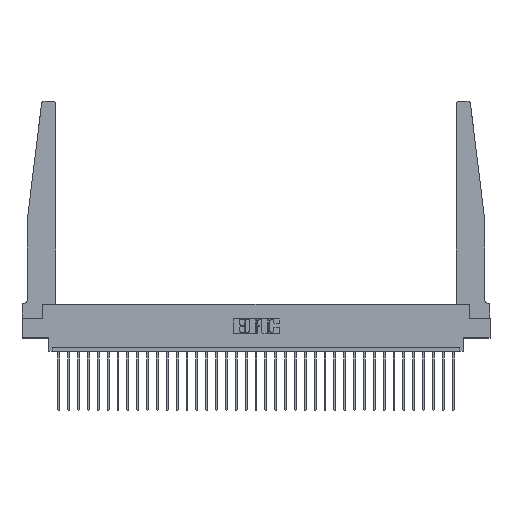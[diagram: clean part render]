
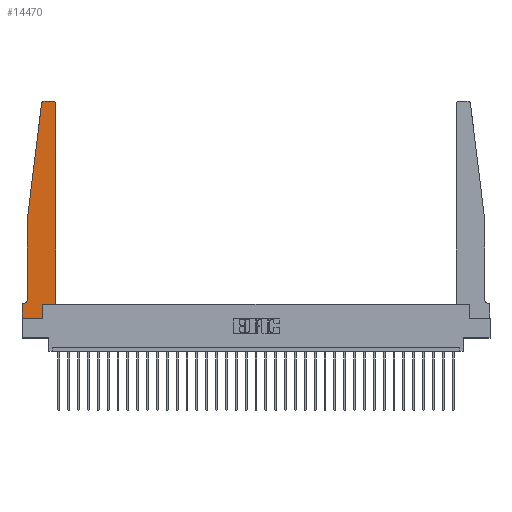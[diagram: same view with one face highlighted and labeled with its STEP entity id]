
A CAD part, top view. The second image highlights one B-rep face of the part: STEP entity #14470.
In plain terms, the highlighted planar face has unit normal (0, 0, 1).
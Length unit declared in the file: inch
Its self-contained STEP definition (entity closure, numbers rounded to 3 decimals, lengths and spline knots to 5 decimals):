
#335 = LINE ( 'NONE', #29155, #5157 ) ;
#478 = VECTOR ( 'NONE', #7500, 39.37008 ) ;
#1019 = VERTEX_POINT ( 'NONE', #19971 ) ;
#2128 = AXIS2_PLACEMENT_3D ( 'NONE', #2731, #24211, #10198 ) ;
#2588 = VERTEX_POINT ( 'NONE', #17972 ) ;
#2600 = DIRECTION ( 'NONE',  ( 0., 0., 1. ) ) ;
#2729 = CARTESIAN_POINT ( 'NONE',  ( 0.425, 0.18, 0.37 ) ) ;
#2731 = CARTESIAN_POINT ( 'NONE',  ( 0.015, 0.2375, 0.37 ) ) ;
#3383 = CARTESIAN_POINT ( 'NONE',  ( 0., 0., 0.37 ) ) ;
#3421 = VECTOR ( 'NONE', #9044, 39.37008 ) ;
#3777 = CARTESIAN_POINT ( 'NONE',  ( 0., 0., 0.37 ) ) ;
#4061 = DIRECTION ( 'NONE',  ( 0., -1., 0. ) ) ;
#4293 = LINE ( 'NONE', #29822, #13118 ) ;
#4560 = EDGE_CURVE ( 'NONE', #19507, #29272, #4293, .T. ) ;
#5157 = VECTOR ( 'NONE', #5846, 39.37008 ) ;
#5846 = DIRECTION ( 'NONE',  ( 0., 1., 0. ) ) ;
#5868 = EDGE_CURVE ( 'NONE', #1019, #19081, #28846, .T. ) ;
#5870 = AXIS2_PLACEMENT_3D ( 'NONE', #26339, #17080, #26533 ) ;
#6393 = EDGE_CURVE ( 'NONE', #19081, #13151, #6403, .T. ) ;
#6403 = LINE ( 'NONE', #25717, #3421 ) ;
#7042 = FACE_OUTER_BOUND ( 'NONE', #27884, .T. ) ;
#7092 = ORIENTED_EDGE ( 'NONE', *, *, #30292, .T. ) ;
#7118 = VECTOR ( 'NONE', #29553, 39.37008 ) ;
#7170 = VERTEX_POINT ( 'NONE', #22088 ) ;
#7500 = DIRECTION ( 'NONE',  ( -0.122, -0.992, 0. ) ) ;
#9044 = DIRECTION ( 'NONE',  ( -1., 0., 0. ) ) ;
#9085 = VECTOR ( 'NONE', #27528, 39.37008 ) ;
#9209 = CARTESIAN_POINT ( 'NONE',  ( 0.425, 0.18, 0.37 ) ) ;
#9689 = DIRECTION ( 'NONE',  ( 1., 0., 0. ) ) ;
#10198 = DIRECTION ( 'NONE',  ( -1., 0., 0. ) ) ;
#10376 = ORIENTED_EDGE ( 'NONE', *, *, #4560, .T. ) ;
#10583 = CIRCLE ( 'NONE', #14198, 0.03 ) ;
#10783 = CARTESIAN_POINT ( 'NONE',  ( 0.395, 2.75, 0.37 ) ) ;
#11486 = CARTESIAN_POINT ( 'NONE',  ( 0., 0., 0.37 ) ) ;
#11532 = LINE ( 'NONE', #15961, #18524 ) ;
#11783 = DIRECTION ( 'NONE',  ( 1., 0., 0. ) ) ;
#11981 = CARTESIAN_POINT ( 'NONE',  ( 0.395, 2.72, 0.37 ) ) ;
#12432 = VERTEX_POINT ( 'NONE', #9209 ) ;
#12606 = LINE ( 'NONE', #20045, #7118 ) ;
#13028 = EDGE_CURVE ( 'NONE', #2588, #16459, #335, .T. ) ;
#13118 = VECTOR ( 'NONE', #18357, 39.37008 ) ;
#13151 = VERTEX_POINT ( 'NONE', #30263 ) ;
#13926 = VERTEX_POINT ( 'NONE', #3777 ) ;
#14198 = AXIS2_PLACEMENT_3D ( 'NONE', #11981, #2600, #11783 ) ;
#14470 = ADVANCED_FACE ( 'NONE', ( #7042 ), #17662, .T. ) ;
#14613 = VECTOR ( 'NONE', #9689, 39.37008 ) ;
#14833 = VERTEX_POINT ( 'NONE', #28486 ) ;
#15491 = DIRECTION ( 'NONE',  ( 1., 0., 0. ) ) ;
#15695 = CARTESIAN_POINT ( 'NONE',  ( 0., 0.1875, 0.37 ) ) ;
#15961 = CARTESIAN_POINT ( 'NONE',  ( 0.425, 0.18, 0.37 ) ) ;
#16459 = VERTEX_POINT ( 'NONE', #22634 ) ;
#16899 = ORIENTED_EDGE ( 'NONE', *, *, #5868, .T. ) ;
#17080 = DIRECTION ( 'NONE',  ( 0., 0., 1. ) ) ;
#17412 = EDGE_CURVE ( 'NONE', #16459, #12432, #25961, .T. ) ;
#17662 = PLANE ( 'NONE',  #23762 ) ;
#17806 = CIRCLE ( 'NONE', #5870, 0.03 ) ;
#17830 = EDGE_CURVE ( 'NONE', #13151, #13926, #22650, .T. ) ;
#17872 = EDGE_CURVE ( 'NONE', #14833, #19507, #10583, .T. ) ;
#17972 = CARTESIAN_POINT ( 'NONE',  ( 0.2605, 0., 0.37 ) ) ;
#18357 = DIRECTION ( 'NONE',  ( -1., 0., 0. ) ) ;
#18524 = VECTOR ( 'NONE', #30218, 39.37008 ) ;
#18651 = VECTOR ( 'NONE', #4061, 39.37008 ) ;
#18838 = CARTESIAN_POINT ( 'NONE',  ( 0.015, 0.1875, 0.37 ) ) ;
#19044 = EDGE_CURVE ( 'NONE', #7170, #26273, #24016, .T. ) ;
#19081 = VERTEX_POINT ( 'NONE', #18838 ) ;
#19507 = VERTEX_POINT ( 'NONE', #10783 ) ;
#19910 = DIRECTION ( 'NONE',  ( 0., 0., 1. ) ) ;
#19971 = CARTESIAN_POINT ( 'NONE',  ( 0.065, 0.2375, 0.37 ) ) ;
#20045 = CARTESIAN_POINT ( 'NONE',  ( 0.065, 1.25, 0.37 ) ) ;
#20674 = ORIENTED_EDGE ( 'NONE', *, *, #6393, .T. ) ;
#21165 = ORIENTED_EDGE ( 'NONE', *, *, #13028, .T. ) ;
#21500 = ORIENTED_EDGE ( 'NONE', *, *, #19044, .T. ) ;
#22088 = CARTESIAN_POINT ( 'NONE',  ( 0.24675, 2.72367, 0.37 ) ) ;
#22130 = ORIENTED_EDGE ( 'NONE', *, *, #17412, .T. ) ;
#22634 = CARTESIAN_POINT ( 'NONE',  ( 0.2605, 0.18, 0.37 ) ) ;
#22650 = LINE ( 'NONE', #11486, #18651 ) ;
#22663 = LINE ( 'NONE', #3383, #9085 ) ;
#23080 = ORIENTED_EDGE ( 'NONE', *, *, #25417, .T. ) ;
#23214 = ORIENTED_EDGE ( 'NONE', *, *, #28178, .T. ) ;
#23464 = CARTESIAN_POINT ( 'NONE',  ( 0.065, 1.25, 0.37 ) ) ;
#23710 = CARTESIAN_POINT ( 'NONE',  ( 0.065, 1.25, 0.37 ) ) ;
#23721 = ORIENTED_EDGE ( 'NONE', *, *, #25341, .T. ) ;
#23762 = AXIS2_PLACEMENT_3D ( 'NONE', #15695, #19910, #15491 ) ;
#24016 = LINE ( 'NONE', #23710, #478 ) ;
#24211 = DIRECTION ( 'NONE',  ( 0., 0., -1. ) ) ;
#24323 = ORIENTED_EDGE ( 'NONE', *, *, #17830, .T. ) ;
#25341 = EDGE_CURVE ( 'NONE', #29272, #7170, #17806, .T. ) ;
#25417 = EDGE_CURVE ( 'NONE', #26273, #1019, #12606, .T. ) ;
#25570 = ORIENTED_EDGE ( 'NONE', *, *, #17872, .T. ) ;
#25717 = CARTESIAN_POINT ( 'NONE',  ( 0.065, 0.1875, 0.37 ) ) ;
#25961 = LINE ( 'NONE', #2729, #14613 ) ;
#26273 = VERTEX_POINT ( 'NONE', #23464 ) ;
#26339 = CARTESIAN_POINT ( 'NONE',  ( 0.27653, 2.72, 0.37 ) ) ;
#26533 = DIRECTION ( 'NONE',  ( 1., 0., 0. ) ) ;
#26928 = CARTESIAN_POINT ( 'NONE',  ( 0.27653, 2.75, 0.37 ) ) ;
#27528 = DIRECTION ( 'NONE',  ( 1., 0., 0. ) ) ;
#27884 = EDGE_LOOP ( 'NONE', ( #10376, #23721, #21500, #23080, #16899, #20674, #24323, #23214, #21165, #22130, #7092, #25570 ) ) ;
#28178 = EDGE_CURVE ( 'NONE', #13926, #2588, #22663, .T. ) ;
#28486 = CARTESIAN_POINT ( 'NONE',  ( 0.425, 2.72, 0.37 ) ) ;
#28846 = CIRCLE ( 'NONE', #2128, 0.05 ) ;
#29155 = CARTESIAN_POINT ( 'NONE',  ( 0.2605, 0.18, 0.37 ) ) ;
#29272 = VERTEX_POINT ( 'NONE', #26928 ) ;
#29553 = DIRECTION ( 'NONE',  ( 0., -1., 0. ) ) ;
#29822 = CARTESIAN_POINT ( 'NONE',  ( 0.25, 2.75, 0.37 ) ) ;
#30218 = DIRECTION ( 'NONE',  ( 0., 1., 0. ) ) ;
#30263 = CARTESIAN_POINT ( 'NONE',  ( 0., 0.1875, 0.37 ) ) ;
#30292 = EDGE_CURVE ( 'NONE', #12432, #14833, #11532, .T. ) ;
